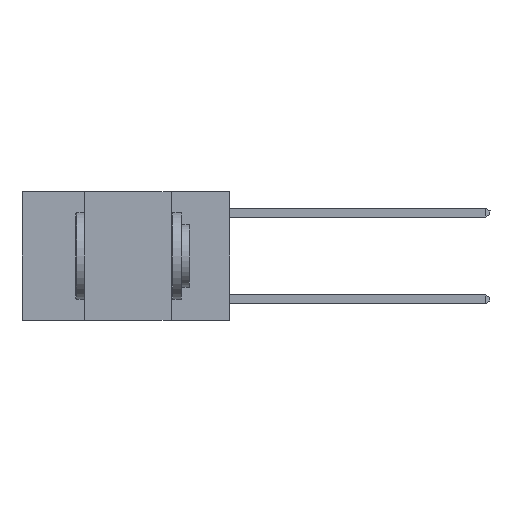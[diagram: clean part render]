
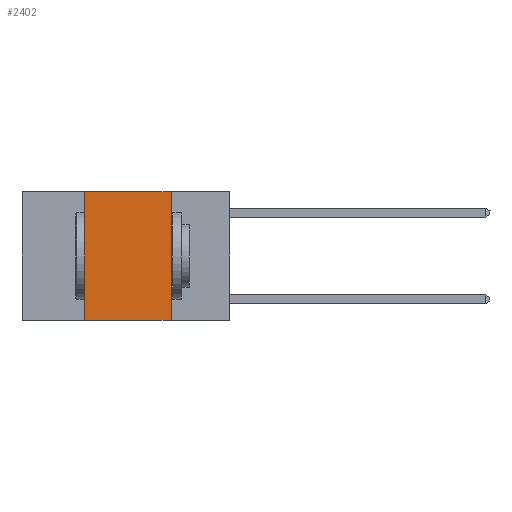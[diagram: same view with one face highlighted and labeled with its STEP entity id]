
A CAD part, left-side view. The second image highlights one B-rep face of the part: STEP entity #2402.
In plain terms, the highlighted planar face has unit normal (-1, 0, 0).
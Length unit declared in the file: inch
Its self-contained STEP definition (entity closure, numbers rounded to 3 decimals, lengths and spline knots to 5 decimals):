
#743 = EDGE_CURVE ( 'NONE', #6149, #4969, #1821, .T. ) ;
#774 = AXIS2_PLACEMENT_3D ( 'NONE', #3686, #8673, #2367 ) ;
#1107 = EDGE_CURVE ( 'NONE', #6149, #8424, #3663, .T. ) ;
#1821 = LINE ( 'NONE', #10455, #3799 ) ;
#2367 = DIRECTION ( 'NONE',  ( 0., 0., -1. ) ) ;
#2402 = ADVANCED_FACE ( 'NONE', ( #5730 ), #3321, .F. ) ;
#2464 = LINE ( 'NONE', #4559, #4705 ) ;
#3321 = PLANE ( 'NONE',  #774 ) ;
#3663 = LINE ( 'NONE', #10077, #7510 ) ;
#3686 = CARTESIAN_POINT ( 'NONE',  ( 0., 0.6, 0. ) ) ;
#3799 = VECTOR ( 'NONE', #9850, 39.37008 ) ;
#4329 = CARTESIAN_POINT ( 'NONE',  ( 0., 0.17, 0. ) ) ;
#4559 = CARTESIAN_POINT ( 'NONE',  ( 0., 0.6, 0. ) ) ;
#4569 = CARTESIAN_POINT ( 'NONE',  ( 0., 0.17, -0.37 ) ) ;
#4705 = VECTOR ( 'NONE', #6999, 39.37008 ) ;
#4717 = EDGE_CURVE ( 'NONE', #8842, #4969, #5415, .T. ) ;
#4969 = VERTEX_POINT ( 'NONE', #4569 ) ;
#5035 = DIRECTION ( 'NONE',  ( 0., 0., -1. ) ) ;
#5320 = ORIENTED_EDGE ( 'NONE', *, *, #7323, .F. ) ;
#5415 = LINE ( 'NONE', #9815, #9421 ) ;
#5730 = FACE_OUTER_BOUND ( 'NONE', #7065, .T. ) ;
#5963 = ORIENTED_EDGE ( 'NONE', *, *, #743, .T. ) ;
#6149 = VERTEX_POINT ( 'NONE', #7687 ) ;
#6285 = ORIENTED_EDGE ( 'NONE', *, *, #1107, .F. ) ;
#6409 = ORIENTED_EDGE ( 'NONE', *, *, #4717, .F. ) ;
#6999 = DIRECTION ( 'NONE',  ( 0., -1., 0. ) ) ;
#7065 = EDGE_LOOP ( 'NONE', ( #6409, #5320, #6285, #5963 ) ) ;
#7323 = EDGE_CURVE ( 'NONE', #8424, #8842, #2464, .T. ) ;
#7510 = VECTOR ( 'NONE', #9997, 39.37008 ) ;
#7687 = CARTESIAN_POINT ( 'NONE',  ( 0., 0.42, -0.37 ) ) ;
#8424 = VERTEX_POINT ( 'NONE', #8603 ) ;
#8603 = CARTESIAN_POINT ( 'NONE',  ( 0., 0.42, 0. ) ) ;
#8673 = DIRECTION ( 'NONE',  ( 1., 0., 0. ) ) ;
#8842 = VERTEX_POINT ( 'NONE', #4329 ) ;
#9421 = VECTOR ( 'NONE', #5035, 39.37008 ) ;
#9815 = CARTESIAN_POINT ( 'NONE',  ( 0., 0.17, 0. ) ) ;
#9850 = DIRECTION ( 'NONE',  ( 0., -1., 0. ) ) ;
#9997 = DIRECTION ( 'NONE',  ( 0., 0., 1. ) ) ;
#10077 = CARTESIAN_POINT ( 'NONE',  ( 0., 0.42, 0. ) ) ;
#10455 = CARTESIAN_POINT ( 'NONE',  ( 0., 0.6, -0.37 ) ) ;
